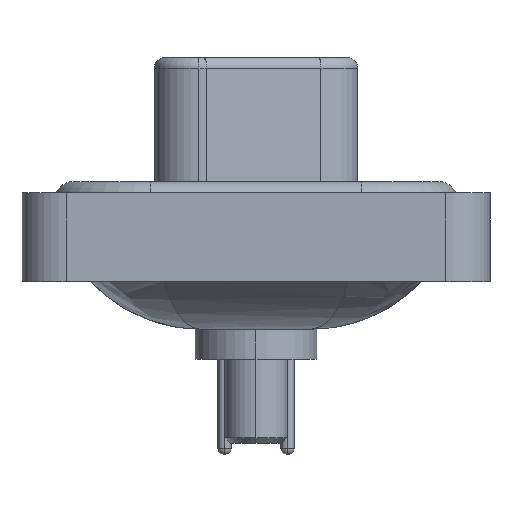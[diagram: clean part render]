
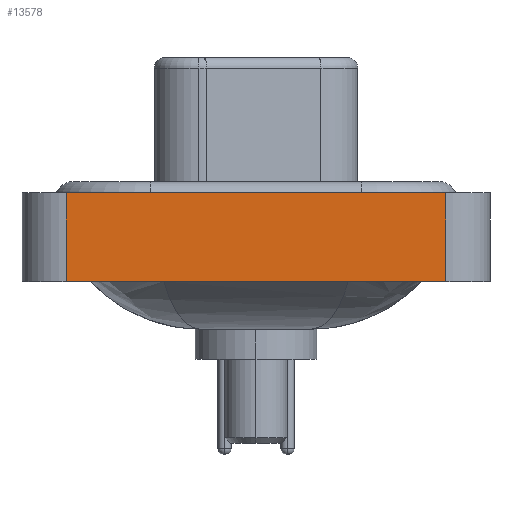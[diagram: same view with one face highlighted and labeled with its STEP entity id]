
A CAD part, left-side view. The second image highlights one B-rep face of the part: STEP entity #13578.
In plain terms, the highlighted planar face has unit normal (-1, 0, 0).
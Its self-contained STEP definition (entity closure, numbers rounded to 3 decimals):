
#397 = ORIENTED_EDGE ( 'NONE', *, *, #7872, .F. ) ;
#635 = VECTOR ( 'NONE', #18955, 1000. ) ;
#1215 = EDGE_CURVE ( 'NONE', #6859, #11990, #6518, .T. ) ;
#1553 = DIRECTION ( 'NONE',  ( 0., 0., 1. ) ) ;
#2170 = CARTESIAN_POINT ( 'NONE',  ( -7.35, -8.55, 0.4 ) ) ;
#2512 = VERTEX_POINT ( 'NONE', #18779 ) ;
#3600 = ORIENTED_EDGE ( 'NONE', *, *, #17634, .F. ) ;
#4263 = CARTESIAN_POINT ( 'NONE',  ( -7.35, -8.55, -3.6 ) ) ;
#4955 = DIRECTION ( 'NONE',  ( 0., 0., 1. ) ) ;
#5507 = AXIS2_PLACEMENT_3D ( 'NONE', #16181, #14292, #4955 ) ;
#6187 = LINE ( 'NONE', #12579, #635 ) ;
#6327 = ORIENTED_EDGE ( 'NONE', *, *, #13348, .T. ) ;
#6518 = LINE ( 'NONE', #10997, #18415 ) ;
#6859 = VERTEX_POINT ( 'NONE', #4263 ) ;
#7756 = ORIENTED_EDGE ( 'NONE', *, *, #1215, .T. ) ;
#7872 = EDGE_CURVE ( 'NONE', #2512, #11990, #6187, .T. ) ;
#8027 = LINE ( 'NONE', #12949, #15880 ) ;
#9671 = LINE ( 'NONE', #15985, #17515 ) ;
#10280 = EDGE_LOOP ( 'NONE', ( #7756, #397, #3600, #6327 ) ) ;
#10997 = CARTESIAN_POINT ( 'NONE',  ( -7.35, -8.55, -3.6 ) ) ;
#11020 = CARTESIAN_POINT ( 'NONE',  ( -7.35, 8.55, -3.6 ) ) ;
#11105 = DIRECTION ( 'NONE',  ( 0., 0., 1. ) ) ;
#11990 = VERTEX_POINT ( 'NONE', #2170 ) ;
#12579 = CARTESIAN_POINT ( 'NONE',  ( -7.35, -8.55, 0.4 ) ) ;
#12949 = CARTESIAN_POINT ( 'NONE',  ( -7.35, -8.55, -3.6 ) ) ;
#13348 = EDGE_CURVE ( 'NONE', #18957, #6859, #8027, .T. ) ;
#13578 = ADVANCED_FACE ( 'NONE', ( #18991 ), #15973, .T. ) ;
#14292 = DIRECTION ( 'NONE',  ( -1., 0., 0. ) ) ;
#14407 = DIRECTION ( 'NONE',  ( 0., -1., 0. ) ) ;
#15880 = VECTOR ( 'NONE', #14407, 1000. ) ;
#15973 = PLANE ( 'NONE',  #5507 ) ;
#15985 = CARTESIAN_POINT ( 'NONE',  ( -7.35, 8.55, -3.6 ) ) ;
#16181 = CARTESIAN_POINT ( 'NONE',  ( -7.35, -8.55, -3.6 ) ) ;
#17515 = VECTOR ( 'NONE', #1553, 1000. ) ;
#17634 = EDGE_CURVE ( 'NONE', #18957, #2512, #9671, .T. ) ;
#18415 = VECTOR ( 'NONE', #11105, 1000. ) ;
#18779 = CARTESIAN_POINT ( 'NONE',  ( -7.35, 8.55, 0.4 ) ) ;
#18955 = DIRECTION ( 'NONE',  ( 0., -1., 0. ) ) ;
#18957 = VERTEX_POINT ( 'NONE', #11020 ) ;
#18991 = FACE_OUTER_BOUND ( 'NONE', #10280, .T. ) ;
